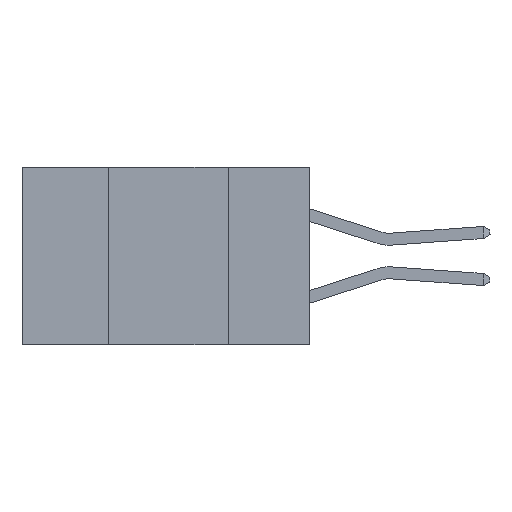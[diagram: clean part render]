
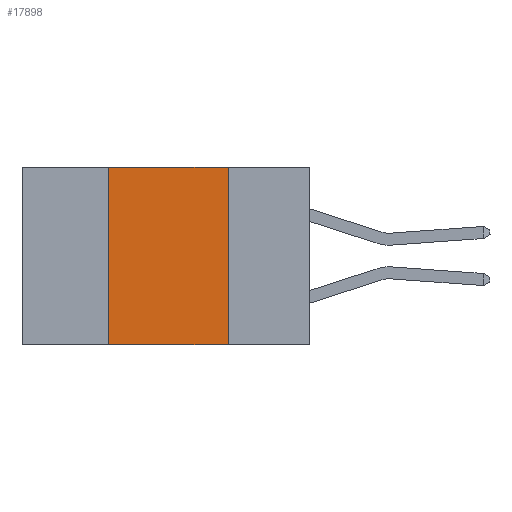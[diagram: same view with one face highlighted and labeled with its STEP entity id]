
A CAD part, left-side view. The second image highlights one B-rep face of the part: STEP entity #17898.
In plain terms, the highlighted planar face has unit normal (-1, 0, 0).
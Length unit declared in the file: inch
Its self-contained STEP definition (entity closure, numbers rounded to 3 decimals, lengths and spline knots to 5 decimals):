
#18 = ORIENTED_EDGE ( 'NONE', *, *, #13415, .F. ) ;
#1305 = FACE_OUTER_BOUND ( 'NONE', #10604, .T. ) ;
#1711 = LINE ( 'NONE', #12365, #5123 ) ;
#3060 = CARTESIAN_POINT ( 'NONE',  ( 0., 0.17, -0.37 ) ) ;
#4655 = DIRECTION ( 'NONE',  ( 0., -1., 0. ) ) ;
#5123 = VECTOR ( 'NONE', #4655, 39.37008 ) ;
#6085 = EDGE_CURVE ( 'NONE', #21413, #13691, #1711, .T. ) ;
#6230 = ORIENTED_EDGE ( 'NONE', *, *, #18897, .F. ) ;
#7164 = LINE ( 'NONE', #10079, #13340 ) ;
#7594 = CARTESIAN_POINT ( 'NONE',  ( 0., 0.42, 0. ) ) ;
#7916 = CARTESIAN_POINT ( 'NONE',  ( 0., 0.6, 0. ) ) ;
#9786 = ORIENTED_EDGE ( 'NONE', *, *, #20359, .F. ) ;
#10079 = CARTESIAN_POINT ( 'NONE',  ( 0., 0.17, 0. ) ) ;
#10187 = CARTESIAN_POINT ( 'NONE',  ( 0., 0.42, 0. ) ) ;
#10204 = VECTOR ( 'NONE', #11632, 39.37008 ) ;
#10535 = ORIENTED_EDGE ( 'NONE', *, *, #6085, .T. ) ;
#10604 = EDGE_LOOP ( 'NONE', ( #6230, #18, #9786, #10535 ) ) ;
#11632 = DIRECTION ( 'NONE',  ( 0., -1., 0. ) ) ;
#12365 = CARTESIAN_POINT ( 'NONE',  ( 0., 0.6, -0.37 ) ) ;
#13340 = VECTOR ( 'NONE', #21962, 39.37008 ) ;
#13415 = EDGE_CURVE ( 'NONE', #18667, #14074, #24402, .T. ) ;
#13601 = PLANE ( 'NONE',  #20105 ) ;
#13691 = VERTEX_POINT ( 'NONE', #3060 ) ;
#13834 = CARTESIAN_POINT ( 'NONE',  ( 0., 0.17, 0. ) ) ;
#14074 = VERTEX_POINT ( 'NONE', #13834 ) ;
#15454 = VECTOR ( 'NONE', #25328, 39.37008 ) ;
#17596 = LINE ( 'NONE', #7594, #15454 ) ;
#17898 = ADVANCED_FACE ( 'NONE', ( #1305 ), #13601, .F. ) ;
#18667 = VERTEX_POINT ( 'NONE', #10187 ) ;
#18897 = EDGE_CURVE ( 'NONE', #14074, #13691, #7164, .T. ) ;
#19008 = CARTESIAN_POINT ( 'NONE',  ( 0., 0.42, -0.37 ) ) ;
#20105 = AXIS2_PLACEMENT_3D ( 'NONE', #25466, #23670, #21850 ) ;
#20359 = EDGE_CURVE ( 'NONE', #21413, #18667, #17596, .T. ) ;
#21413 = VERTEX_POINT ( 'NONE', #19008 ) ;
#21850 = DIRECTION ( 'NONE',  ( 0., 0., -1. ) ) ;
#21962 = DIRECTION ( 'NONE',  ( 0., 0., -1. ) ) ;
#23670 = DIRECTION ( 'NONE',  ( 1., 0., 0. ) ) ;
#24402 = LINE ( 'NONE', #7916, #10204 ) ;
#25328 = DIRECTION ( 'NONE',  ( 0., 0., 1. ) ) ;
#25466 = CARTESIAN_POINT ( 'NONE',  ( 0., 0.6, 0. ) ) ;
